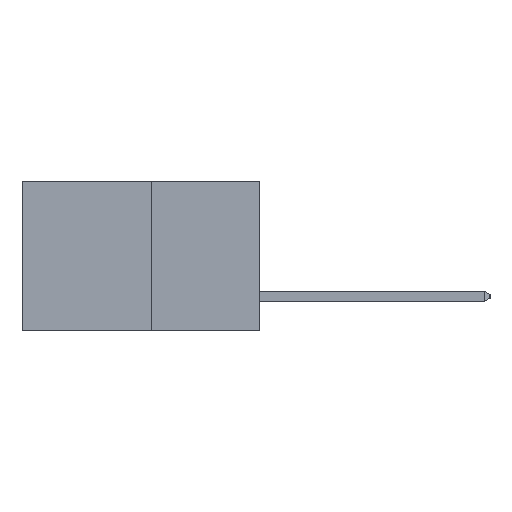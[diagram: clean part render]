
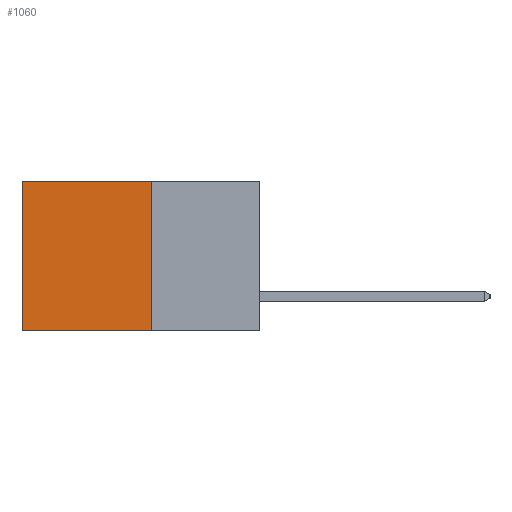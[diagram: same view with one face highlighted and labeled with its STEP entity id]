
A CAD part, left-side view. The second image highlights one B-rep face of the part: STEP entity #1060.
In plain terms, the highlighted planar face has unit normal (-1, 0, 0).
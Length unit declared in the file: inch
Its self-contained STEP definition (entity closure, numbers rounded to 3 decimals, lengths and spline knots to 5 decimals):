
#719 = VERTEX_POINT ( 'NONE', #3279 ) ;
#1060 = ADVANCED_FACE ( 'NONE', ( #12732 ), #9731, .F. ) ;
#1514 = CARTESIAN_POINT ( 'NONE',  ( 0.277, 0.59, 0. ) ) ;
#2005 = VECTOR ( 'NONE', #9718, 39.37008 ) ;
#2112 = ORIENTED_EDGE ( 'NONE', *, *, #8805, .T. ) ;
#2155 = DIRECTION ( 'NONE',  ( 0., 0., -1. ) ) ;
#2514 = ORIENTED_EDGE ( 'NONE', *, *, #4746, .F. ) ;
#3279 = CARTESIAN_POINT ( 'NONE',  ( 0.277, 0.59, -0.37 ) ) ;
#4182 = DIRECTION ( 'NONE',  ( 0., 1., 0. ) ) ;
#4362 = CARTESIAN_POINT ( 'NONE',  ( 0.277, 0.27, -0.37 ) ) ;
#4746 = EDGE_CURVE ( 'NONE', #11323, #719, #6395, .T. ) ;
#5088 = LINE ( 'NONE', #9745, #2005 ) ;
#5268 = LINE ( 'NONE', #14324, #13774 ) ;
#6395 = LINE ( 'NONE', #4362, #14507 ) ;
#6526 = ORIENTED_EDGE ( 'NONE', *, *, #9223, .F. ) ;
#6982 = CARTESIAN_POINT ( 'NONE',  ( 0.277, 0.27, -0.37 ) ) ;
#7001 = DIRECTION ( 'NONE',  ( 0., 0., -1. ) ) ;
#7388 = AXIS2_PLACEMENT_3D ( 'NONE', #14150, #13223, #2155 ) ;
#7436 = VERTEX_POINT ( 'NONE', #12114 ) ;
#8159 = EDGE_CURVE ( 'NONE', #7436, #11190, #5268, .T. ) ;
#8541 = VECTOR ( 'NONE', #7001, 39.37008 ) ;
#8805 = EDGE_CURVE ( 'NONE', #11190, #719, #5088, .T. ) ;
#9223 = EDGE_CURVE ( 'NONE', #7436, #11323, #11844, .T. ) ;
#9718 = DIRECTION ( 'NONE',  ( 0., 0., -1. ) ) ;
#9731 = PLANE ( 'NONE',  #7388 ) ;
#9745 = CARTESIAN_POINT ( 'NONE',  ( 0.277, 0.59, -0.37 ) ) ;
#10717 = EDGE_LOOP ( 'NONE', ( #2112, #2514, #6526, #12471 ) ) ;
#11190 = VERTEX_POINT ( 'NONE', #1514 ) ;
#11323 = VERTEX_POINT ( 'NONE', #11852 ) ;
#11844 = LINE ( 'NONE', #6982, #8541 ) ;
#11852 = CARTESIAN_POINT ( 'NONE',  ( 0.277, 0.27, -0.37 ) ) ;
#12114 = CARTESIAN_POINT ( 'NONE',  ( 0.277, 0.27, 0. ) ) ;
#12471 = ORIENTED_EDGE ( 'NONE', *, *, #8159, .T. ) ;
#12732 = FACE_OUTER_BOUND ( 'NONE', #10717, .T. ) ;
#13223 = DIRECTION ( 'NONE',  ( 1., 0., 0. ) ) ;
#13774 = VECTOR ( 'NONE', #14104, 39.37008 ) ;
#14104 = DIRECTION ( 'NONE',  ( 0., 1., 0. ) ) ;
#14150 = CARTESIAN_POINT ( 'NONE',  ( 0.277, 0.27, -0.37 ) ) ;
#14324 = CARTESIAN_POINT ( 'NONE',  ( 0.277, 0.27, 0. ) ) ;
#14507 = VECTOR ( 'NONE', #4182, 39.37008 ) ;
